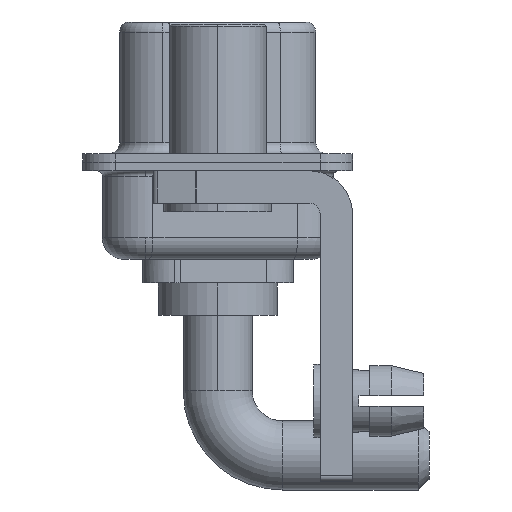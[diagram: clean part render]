
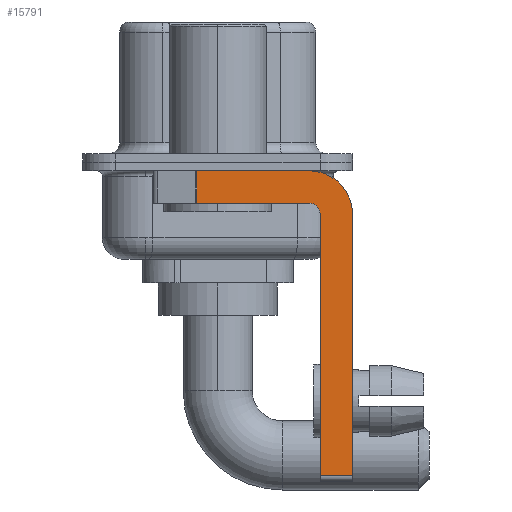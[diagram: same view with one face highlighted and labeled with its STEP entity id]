
A CAD part, left-side view. The second image highlights one B-rep face of the part: STEP entity #15791.
In plain terms, the highlighted planar face has unit normal (-1, 0, 0).
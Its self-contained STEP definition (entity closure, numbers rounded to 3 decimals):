
#142 = DIRECTION ( 'NONE',  ( 0., 0., -1. ) ) ;
#258 = LINE ( 'NONE', #13173, #4025 ) ;
#525 = EDGE_CURVE ( 'NONE', #10421, #4951, #16370, .T. ) ;
#967 = CARTESIAN_POINT ( 'NONE',  ( -2.9, -4.25, -1.9 ) ) ;
#1028 = CIRCLE ( 'NONE', #3407, 2. ) ;
#1218 = CARTESIAN_POINT ( 'NONE',  ( -2.9, -6.25, -2.4 ) ) ;
#1450 = DIRECTION ( 'NONE',  ( 0., 0., 1. ) ) ;
#1931 = VERTEX_POINT ( 'NONE', #13145 ) ;
#2850 = ORIENTED_EDGE ( 'NONE', *, *, #8990, .F. ) ;
#2874 = DIRECTION ( 'NONE',  ( 0., -1., 0. ) ) ;
#2945 = DIRECTION ( 'NONE',  ( 0., 0., -1. ) ) ;
#3407 = AXIS2_PLACEMENT_3D ( 'NONE', #11344, #14347, #5986 ) ;
#3474 = VERTEX_POINT ( 'NONE', #14518 ) ;
#3780 = CARTESIAN_POINT ( 'NONE',  ( -2.9, -4.25, -2.4 ) ) ;
#3856 = EDGE_LOOP ( 'NONE', ( #9212, #16060, #17349, #4263, #2850, #12547, #5602, #8996 ) ) ;
#3902 = EDGE_CURVE ( 'NONE', #18408, #7479, #12069, .T. ) ;
#3998 = VECTOR ( 'NONE', #142, 1000. ) ;
#4025 = VECTOR ( 'NONE', #10171, 1000. ) ;
#4052 = DIRECTION ( 'NONE',  ( 1., 0., 0. ) ) ;
#4235 = LINE ( 'NONE', #4324, #15848 ) ;
#4263 = ORIENTED_EDGE ( 'NONE', *, *, #525, .F. ) ;
#4324 = CARTESIAN_POINT ( 'NONE',  ( -2.9, -6.25, -2.4 ) ) ;
#4951 = VERTEX_POINT ( 'NONE', #967 ) ;
#5106 = CARTESIAN_POINT ( 'NONE',  ( -2.9, -4.75, -2.4 ) ) ;
#5224 = EDGE_CURVE ( 'NONE', #9869, #7479, #4235, .T. ) ;
#5602 = ORIENTED_EDGE ( 'NONE', *, *, #5224, .F. ) ;
#5986 = DIRECTION ( 'NONE',  ( 0., 0., -1. ) ) ;
#7469 = EDGE_CURVE ( 'NONE', #15536, #1931, #9621, .T. ) ;
#7479 = VERTEX_POINT ( 'NONE', #12975 ) ;
#8601 = CARTESIAN_POINT ( 'NONE',  ( -2.9, -4.75, -14.8 ) ) ;
#8663 = CARTESIAN_POINT ( 'NONE',  ( -2.9, 3., -0.4 ) ) ;
#8990 = EDGE_CURVE ( 'NONE', #18408, #10421, #9993, .T. ) ;
#8996 = ORIENTED_EDGE ( 'NONE', *, *, #17799, .F. ) ;
#9072 = VECTOR ( 'NONE', #2874, 1000. ) ;
#9212 = ORIENTED_EDGE ( 'NONE', *, *, #7469, .F. ) ;
#9621 = LINE ( 'NONE', #8663, #9072 ) ;
#9669 = FACE_OUTER_BOUND ( 'NONE', #3856, .T. ) ;
#9869 = VERTEX_POINT ( 'NONE', #1218 ) ;
#9993 = LINE ( 'NONE', #8601, #16603 ) ;
#10171 = DIRECTION ( 'NONE',  ( 0., 1., 0. ) ) ;
#10265 = DIRECTION ( 'NONE',  ( 0., 0., 1. ) ) ;
#10329 = LINE ( 'NONE', #16068, #3998 ) ;
#10421 = VERTEX_POINT ( 'NONE', #5106 ) ;
#10513 = CARTESIAN_POINT ( 'NONE',  ( -2.9, 0.978, -0.4 ) ) ;
#11289 = AXIS2_PLACEMENT_3D ( 'NONE', #17367, #13143, #1450 ) ;
#11344 = CARTESIAN_POINT ( 'NONE',  ( -2.9, -4.25, -2.4 ) ) ;
#12069 = LINE ( 'NONE', #16194, #13980 ) ;
#12547 = ORIENTED_EDGE ( 'NONE', *, *, #3902, .T. ) ;
#12975 = CARTESIAN_POINT ( 'NONE',  ( -2.9, -6.25, -14.55 ) ) ;
#13143 = DIRECTION ( 'NONE',  ( -1., 0., 0. ) ) ;
#13145 = CARTESIAN_POINT ( 'NONE',  ( -2.9, -4.25, -0.4 ) ) ;
#13173 = CARTESIAN_POINT ( 'NONE',  ( -2.9, -4.25, -1.9 ) ) ;
#13980 = VECTOR ( 'NONE', #14892, 1000. ) ;
#14347 = DIRECTION ( 'NONE',  ( 1., 0., 0. ) ) ;
#14518 = CARTESIAN_POINT ( 'NONE',  ( -2.9, 0.978, -1.9 ) ) ;
#14892 = DIRECTION ( 'NONE',  ( 0., -1., 0. ) ) ;
#15084 = CARTESIAN_POINT ( 'NONE',  ( -2.9, -4.75, -14.55 ) ) ;
#15373 = AXIS2_PLACEMENT_3D ( 'NONE', #3780, #4052, #18319 ) ;
#15390 = PLANE ( 'NONE',  #15373 ) ;
#15445 = EDGE_CURVE ( 'NONE', #15536, #3474, #10329, .T. ) ;
#15536 = VERTEX_POINT ( 'NONE', #10513 ) ;
#15791 = ADVANCED_FACE ( 'NONE', ( #9669 ), #15390, .F. ) ;
#15848 = VECTOR ( 'NONE', #2945, 1000. ) ;
#16060 = ORIENTED_EDGE ( 'NONE', *, *, #15445, .T. ) ;
#16068 = CARTESIAN_POINT ( 'NONE',  ( -2.9, 0.978, -1.9 ) ) ;
#16194 = CARTESIAN_POINT ( 'NONE',  ( -2.9, -4.25, -14.55 ) ) ;
#16370 = CIRCLE ( 'NONE', #11289, 0.5 ) ;
#16603 = VECTOR ( 'NONE', #10265, 1000. ) ;
#17349 = ORIENTED_EDGE ( 'NONE', *, *, #18001, .F. ) ;
#17367 = CARTESIAN_POINT ( 'NONE',  ( -2.9, -4.25, -2.4 ) ) ;
#17799 = EDGE_CURVE ( 'NONE', #1931, #9869, #1028, .T. ) ;
#18001 = EDGE_CURVE ( 'NONE', #4951, #3474, #258, .T. ) ;
#18319 = DIRECTION ( 'NONE',  ( 0., 0., -1. ) ) ;
#18408 = VERTEX_POINT ( 'NONE', #15084 ) ;
